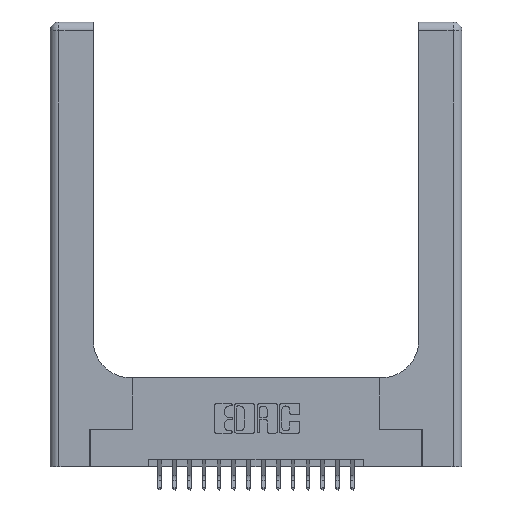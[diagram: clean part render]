
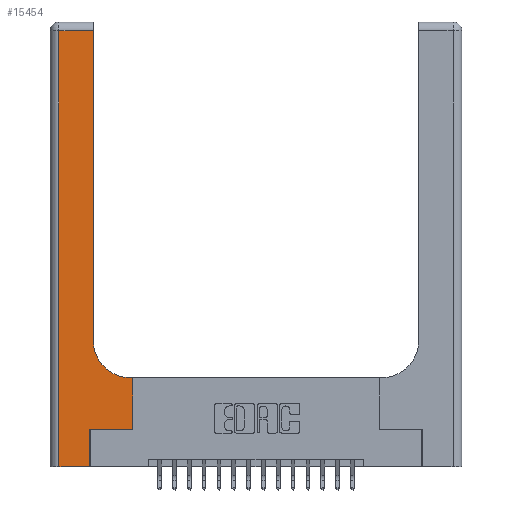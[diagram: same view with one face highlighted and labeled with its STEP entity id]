
A CAD part, top view. The second image highlights one B-rep face of the part: STEP entity #15454.
In plain terms, the highlighted planar face has unit normal (0, 0, 1).
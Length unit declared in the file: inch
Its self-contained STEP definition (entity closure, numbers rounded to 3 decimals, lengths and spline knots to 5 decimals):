
#10 = VERTEX_POINT ( 'NONE', #11574 ) ;
#514 = LINE ( 'NONE', #13420, #16567 ) ;
#564 = CARTESIAN_POINT ( 'NONE',  ( 0.2915, 2.94, 0.37 ) ) ;
#637 = VECTOR ( 'NONE', #9516, 39.37008 ) ;
#1764 = EDGE_CURVE ( 'NONE', #14315, #3060, #6250, .T. ) ;
#1774 = CARTESIAN_POINT ( 'NONE',  ( 0.5585, 0.6, 0.37 ) ) ;
#1870 = CARTESIAN_POINT ( 'NONE',  ( 0.269, 0., 0.37 ) ) ;
#2006 = EDGE_CURVE ( 'NONE', #16878, #18316, #13021, .T. ) ;
#2099 = VECTOR ( 'NONE', #15012, 39.37008 ) ;
#2152 = EDGE_CURVE ( 'NONE', #16800, #10, #2578, .T. ) ;
#2578 = LINE ( 'NONE', #2852, #4767 ) ;
#2852 = CARTESIAN_POINT ( 'NONE',  ( 0.269, 0.25, 0.37 ) ) ;
#3060 = VERTEX_POINT ( 'NONE', #6391 ) ;
#3941 = DIRECTION ( 'NONE',  ( 1., 0., 0. ) ) ;
#4767 = VECTOR ( 'NONE', #6055, 39.37008 ) ;
#4986 = ORIENTED_EDGE ( 'NONE', *, *, #2006, .T. ) ;
#5014 = DIRECTION ( 'NONE',  ( 0., 0., -1. ) ) ;
#5045 = ORIENTED_EDGE ( 'NONE', *, *, #13495, .T. ) ;
#5057 = DIRECTION ( 'NONE',  ( 0., 1., 0. ) ) ;
#5233 = FACE_OUTER_BOUND ( 'NONE', #13531, .T. ) ;
#5541 = LINE ( 'NONE', #1870, #20122 ) ;
#5837 = CARTESIAN_POINT ( 'NONE',  ( 0.5415, 0.6, 0.37 ) ) ;
#5979 = CARTESIAN_POINT ( 'NONE',  ( 0.269, 0.25, 0.37 ) ) ;
#6055 = DIRECTION ( 'NONE',  ( 1., 0., 0. ) ) ;
#6250 = LINE ( 'NONE', #12851, #637 ) ;
#6391 = CARTESIAN_POINT ( 'NONE',  ( 0.06, 0., 0.37 ) ) ;
#6446 = CARTESIAN_POINT ( 'NONE',  ( 0., 3., 0.37 ) ) ;
#6492 = VERTEX_POINT ( 'NONE', #18446 ) ;
#7120 = ORIENTED_EDGE ( 'NONE', *, *, #11496, .T. ) ;
#7494 = CARTESIAN_POINT ( 'NONE',  ( 0., 2.94, 0.37 ) ) ;
#8086 = ORIENTED_EDGE ( 'NONE', *, *, #13453, .T. ) ;
#8356 = CARTESIAN_POINT ( 'NONE',  ( 0.5585, 0.25, 0.37 ) ) ;
#8456 = VECTOR ( 'NONE', #12239, 39.37008 ) ;
#9028 = EDGE_CURVE ( 'NONE', #3060, #6492, #514, .T. ) ;
#9516 = DIRECTION ( 'NONE',  ( 0., -1., 0. ) ) ;
#10305 = VECTOR ( 'NONE', #16170, 39.37008 ) ;
#10414 = ORIENTED_EDGE ( 'NONE', *, *, #13335, .T. ) ;
#11496 = EDGE_CURVE ( 'NONE', #6492, #16800, #5541, .T. ) ;
#11574 = CARTESIAN_POINT ( 'NONE',  ( 0.5585, 0.25, 0.37 ) ) ;
#11620 = CARTESIAN_POINT ( 'NONE',  ( 0.2915, 3., 0.37 ) ) ;
#11988 = ORIENTED_EDGE ( 'NONE', *, *, #15664, .T. ) ;
#12011 = LINE ( 'NONE', #8356, #10305 ) ;
#12239 = DIRECTION ( 'NONE',  ( -1., 0., 0. ) ) ;
#12318 = LINE ( 'NONE', #7494, #8456 ) ;
#12524 = CARTESIAN_POINT ( 'NONE',  ( 0.2915, 0.85, 0.37 ) ) ;
#12851 = CARTESIAN_POINT ( 'NONE',  ( 0.06, 3., 0.37 ) ) ;
#13021 = CIRCLE ( 'NONE', #17378, 0.25 ) ;
#13335 = EDGE_CURVE ( 'NONE', #10, #19779, #12011, .T. ) ;
#13420 = CARTESIAN_POINT ( 'NONE',  ( 0., 0., 0.37 ) ) ;
#13453 = EDGE_CURVE ( 'NONE', #18316, #15587, #17645, .T. ) ;
#13495 = EDGE_CURVE ( 'NONE', #19779, #16878, #15163, .T. ) ;
#13531 = EDGE_LOOP ( 'NONE', ( #8086, #11988, #14456, #18361, #7120, #20002, #10414, #5045, #4986 ) ) ;
#13634 = DIRECTION ( 'NONE',  ( -1., 0., 0. ) ) ;
#13702 = CARTESIAN_POINT ( 'NONE',  ( 0.2915, 0.6, 0.37 ) ) ;
#13994 = CARTESIAN_POINT ( 'NONE',  ( 0.5415, 0.85, 0.37 ) ) ;
#14065 = DIRECTION ( 'NONE',  ( 0., 0., -1. ) ) ;
#14315 = VERTEX_POINT ( 'NONE', #17885 ) ;
#14456 = ORIENTED_EDGE ( 'NONE', *, *, #1764, .T. ) ;
#14671 = VECTOR ( 'NONE', #13634, 39.37008 ) ;
#15012 = DIRECTION ( 'NONE',  ( 0., 1., 0. ) ) ;
#15163 = LINE ( 'NONE', #13702, #14671 ) ;
#15454 = ADVANCED_FACE ( 'NONE', ( #5233 ), #19073, .F. ) ;
#15587 = VERTEX_POINT ( 'NONE', #564 ) ;
#15664 = EDGE_CURVE ( 'NONE', #15587, #14315, #12318, .T. ) ;
#15848 = DIRECTION ( 'NONE',  ( -1., 0., 0. ) ) ;
#16170 = DIRECTION ( 'NONE',  ( 0., 1., 0. ) ) ;
#16567 = VECTOR ( 'NONE', #3941, 39.37008 ) ;
#16800 = VERTEX_POINT ( 'NONE', #5979 ) ;
#16878 = VERTEX_POINT ( 'NONE', #5837 ) ;
#17066 = DIRECTION ( 'NONE',  ( 1., 0., 0. ) ) ;
#17119 = AXIS2_PLACEMENT_3D ( 'NONE', #6446, #5014, #15848 ) ;
#17378 = AXIS2_PLACEMENT_3D ( 'NONE', #13994, #14065, #17066 ) ;
#17645 = LINE ( 'NONE', #11620, #2099 ) ;
#17885 = CARTESIAN_POINT ( 'NONE',  ( 0.06, 2.94, 0.37 ) ) ;
#18316 = VERTEX_POINT ( 'NONE', #12524 ) ;
#18361 = ORIENTED_EDGE ( 'NONE', *, *, #9028, .T. ) ;
#18446 = CARTESIAN_POINT ( 'NONE',  ( 0.269, 0., 0.37 ) ) ;
#19073 = PLANE ( 'NONE',  #17119 ) ;
#19779 = VERTEX_POINT ( 'NONE', #1774 ) ;
#20002 = ORIENTED_EDGE ( 'NONE', *, *, #2152, .T. ) ;
#20122 = VECTOR ( 'NONE', #5057, 39.37008 ) ;
